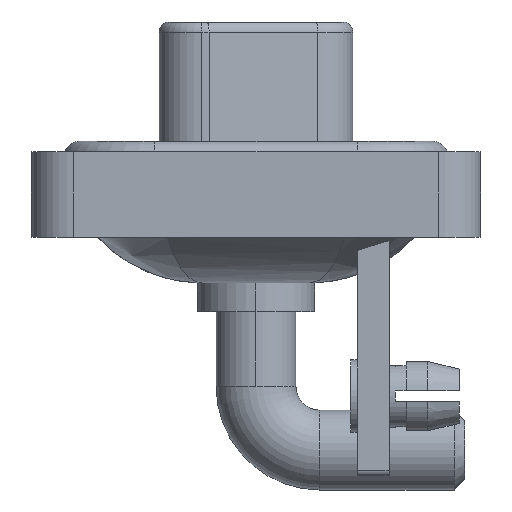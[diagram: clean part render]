
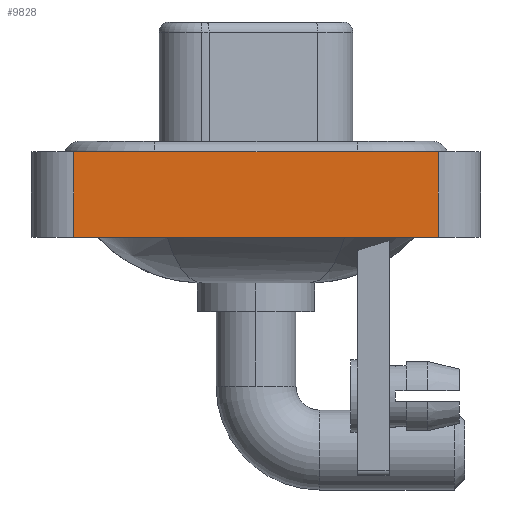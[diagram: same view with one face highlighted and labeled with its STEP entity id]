
A CAD part, left-side view. The second image highlights one B-rep face of the part: STEP entity #9828.
In plain terms, the highlighted planar face has unit normal (-1, 0, 0).
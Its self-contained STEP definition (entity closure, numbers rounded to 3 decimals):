
#70 = EDGE_CURVE ( 'NONE', #4872, #4595, #12164, .T. ) ;
#429 = CARTESIAN_POINT ( 'NONE',  ( -7.3, -8.55, -3.6 ) ) ;
#1263 = LINE ( 'NONE', #7080, #4619 ) ;
#1294 = CARTESIAN_POINT ( 'NONE',  ( -7.3, 8.55, 0.4 ) ) ;
#2089 = FACE_OUTER_BOUND ( 'NONE', #5668, .T. ) ;
#3073 = EDGE_CURVE ( 'NONE', #10098, #4595, #14880, .T. ) ;
#3613 = ORIENTED_EDGE ( 'NONE', *, *, #5622, .F. ) ;
#4595 = VERTEX_POINT ( 'NONE', #4651 ) ;
#4619 = VECTOR ( 'NONE', #14827, 1000. ) ;
#4651 = CARTESIAN_POINT ( 'NONE',  ( -7.3, -8.55, 0.4 ) ) ;
#4853 = DIRECTION ( 'NONE',  ( -1., 0., 0. ) ) ;
#4872 = VERTEX_POINT ( 'NONE', #1294 ) ;
#4909 = DIRECTION ( 'NONE',  ( 0., -1., 0. ) ) ;
#5376 = AXIS2_PLACEMENT_3D ( 'NONE', #13536, #4853, #17646 ) ;
#5622 = EDGE_CURVE ( 'NONE', #13804, #4872, #17961, .T. ) ;
#5668 = EDGE_LOOP ( 'NONE', ( #17136, #14593, #3613, #9179 ) ) ;
#5692 = CARTESIAN_POINT ( 'NONE',  ( -7.3, -8.55, -3.6 ) ) ;
#6611 = VECTOR ( 'NONE', #6694, 1000. ) ;
#6694 = DIRECTION ( 'NONE',  ( 0., 0., 1. ) ) ;
#7080 = CARTESIAN_POINT ( 'NONE',  ( -7.3, -8.55, -3.6 ) ) ;
#7718 = PLANE ( 'NONE',  #5376 ) ;
#8951 = DIRECTION ( 'NONE',  ( 0., 0., 1. ) ) ;
#9179 = ORIENTED_EDGE ( 'NONE', *, *, #13757, .T. ) ;
#9828 = ADVANCED_FACE ( 'NONE', ( #2089 ), #7718, .T. ) ;
#10098 = VERTEX_POINT ( 'NONE', #5692 ) ;
#12164 = LINE ( 'NONE', #17981, #12581 ) ;
#12581 = VECTOR ( 'NONE', #4909, 1000. ) ;
#13536 = CARTESIAN_POINT ( 'NONE',  ( -7.3, -8.55, -3.6 ) ) ;
#13757 = EDGE_CURVE ( 'NONE', #13804, #10098, #1263, .T. ) ;
#13804 = VERTEX_POINT ( 'NONE', #17395 ) ;
#14593 = ORIENTED_EDGE ( 'NONE', *, *, #70, .F. ) ;
#14827 = DIRECTION ( 'NONE',  ( 0., -1., 0. ) ) ;
#14880 = LINE ( 'NONE', #429, #17245 ) ;
#17136 = ORIENTED_EDGE ( 'NONE', *, *, #3073, .T. ) ;
#17245 = VECTOR ( 'NONE', #8951, 1000. ) ;
#17395 = CARTESIAN_POINT ( 'NONE',  ( -7.3, 8.55, -3.6 ) ) ;
#17646 = DIRECTION ( 'NONE',  ( 0., 0., 1. ) ) ;
#17961 = LINE ( 'NONE', #18051, #6611 ) ;
#17981 = CARTESIAN_POINT ( 'NONE',  ( -7.3, -8.55, 0.4 ) ) ;
#18051 = CARTESIAN_POINT ( 'NONE',  ( -7.3, 8.55, -3.6 ) ) ;
